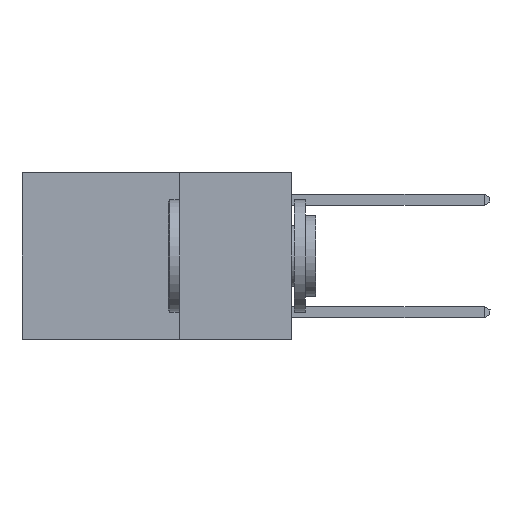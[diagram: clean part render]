
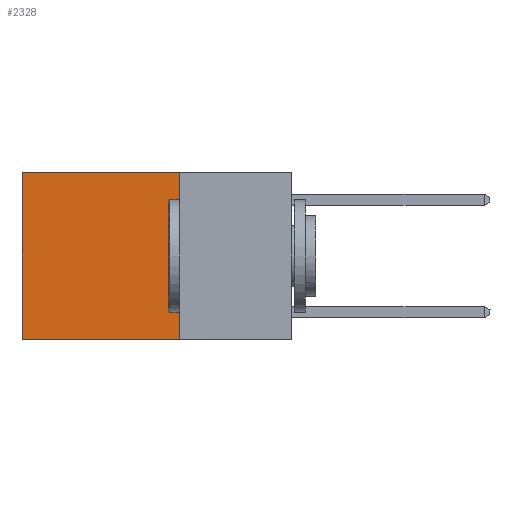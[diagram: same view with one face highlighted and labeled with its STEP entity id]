
A CAD part, left-side view. The second image highlights one B-rep face of the part: STEP entity #2328.
In plain terms, the highlighted planar face has unit normal (-1, 0, 0).
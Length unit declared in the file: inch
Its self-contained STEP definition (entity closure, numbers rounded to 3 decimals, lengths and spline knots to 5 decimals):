
#289 = DIRECTION ( 'NONE',  ( 0., 1., 0. ) ) ;
#374 = LINE ( 'NONE', #8293, #6634 ) ;
#492 = CARTESIAN_POINT ( 'NONE',  ( 0.2625, 0.25, 0. ) ) ;
#734 = AXIS2_PLACEMENT_3D ( 'NONE', #492, #6983, #2185 ) ;
#879 = CARTESIAN_POINT ( 'NONE',  ( 0.2625, 0.6, 0. ) ) ;
#1150 = CARTESIAN_POINT ( 'NONE',  ( 0.2625, 0.25, 0. ) ) ;
#1223 = CARTESIAN_POINT ( 'NONE',  ( 0.2625, 0.6, 0. ) ) ;
#1339 = VERTEX_POINT ( 'NONE', #3534 ) ;
#1756 = ORIENTED_EDGE ( 'NONE', *, *, #2249, .F. ) ;
#1792 = VECTOR ( 'NONE', #9151, 39.37008 ) ;
#2185 = DIRECTION ( 'NONE',  ( 0., 0., -1. ) ) ;
#2219 = EDGE_CURVE ( 'NONE', #1339, #9551, #374, .T. ) ;
#2249 = EDGE_CURVE ( 'NONE', #1339, #2837, #4448, .T. ) ;
#2328 = ADVANCED_FACE ( 'NONE', ( #7193 ), #7679, .F. ) ;
#2487 = ORIENTED_EDGE ( 'NONE', *, *, #2219, .T. ) ;
#2778 = DIRECTION ( 'NONE',  ( 0., 1., 0. ) ) ;
#2796 = CARTESIAN_POINT ( 'NONE',  ( 0.2625, 0.25, -0.37 ) ) ;
#2837 = VERTEX_POINT ( 'NONE', #2796 ) ;
#3534 = CARTESIAN_POINT ( 'NONE',  ( 0.2625, 0.25, 0. ) ) ;
#4448 = LINE ( 'NONE', #1150, #1792 ) ;
#4534 = DIRECTION ( 'NONE',  ( 0., 0., -1. ) ) ;
#5342 = EDGE_LOOP ( 'NONE', ( #5368, #7824, #1756, #2487 ) ) ;
#5368 = ORIENTED_EDGE ( 'NONE', *, *, #9154, .T. ) ;
#6474 = VECTOR ( 'NONE', #289, 39.37008 ) ;
#6634 = VECTOR ( 'NONE', #2778, 39.37008 ) ;
#6958 = VERTEX_POINT ( 'NONE', #7059 ) ;
#6983 = DIRECTION ( 'NONE',  ( 1., 0., 0. ) ) ;
#7059 = CARTESIAN_POINT ( 'NONE',  ( 0.2625, 0.6, -0.37 ) ) ;
#7193 = FACE_OUTER_BOUND ( 'NONE', #5342, .T. ) ;
#7495 = VECTOR ( 'NONE', #4534, 39.37008 ) ;
#7496 = CARTESIAN_POINT ( 'NONE',  ( 0.2625, 0.25, -0.37 ) ) ;
#7679 = PLANE ( 'NONE',  #734 ) ;
#7824 = ORIENTED_EDGE ( 'NONE', *, *, #9085, .F. ) ;
#8293 = CARTESIAN_POINT ( 'NONE',  ( 0.2625, 0.25, 0. ) ) ;
#8475 = LINE ( 'NONE', #7496, #6474 ) ;
#9085 = EDGE_CURVE ( 'NONE', #2837, #6958, #8475, .T. ) ;
#9151 = DIRECTION ( 'NONE',  ( 0., 0., -1. ) ) ;
#9154 = EDGE_CURVE ( 'NONE', #9551, #6958, #9318, .T. ) ;
#9318 = LINE ( 'NONE', #1223, #7495 ) ;
#9551 = VERTEX_POINT ( 'NONE', #879 ) ;
